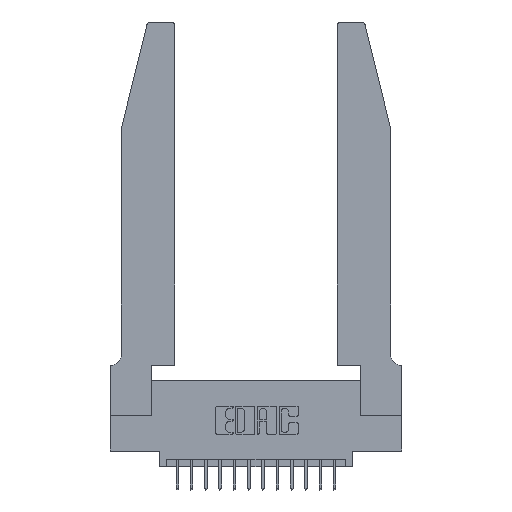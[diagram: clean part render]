
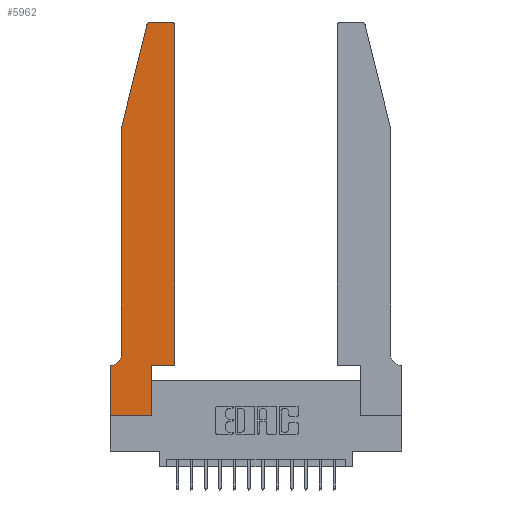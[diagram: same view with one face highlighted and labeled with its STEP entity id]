
A CAD part, top view. The second image highlights one B-rep face of the part: STEP entity #5962.
In plain terms, the highlighted planar face has unit normal (0, 0, 1).
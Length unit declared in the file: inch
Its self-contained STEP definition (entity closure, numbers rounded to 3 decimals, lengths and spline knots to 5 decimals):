
#3 = EDGE_CURVE ( 'NONE', #927, #10412, #13001, .T. ) ;
#71 = LINE ( 'NONE', #13692, #7374 ) ;
#250 = DIRECTION ( 'NONE',  ( -1., 0., 0. ) ) ;
#412 = DIRECTION ( 'NONE',  ( 0., 0., -1. ) ) ;
#456 = CARTESIAN_POINT ( 'NONE',  ( 0.0055, 0.42, 0.37 ) ) ;
#556 = VERTEX_POINT ( 'NONE', #3876 ) ;
#640 = EDGE_CURVE ( 'NONE', #1668, #1718, #12131, .T. ) ;
#649 = EDGE_CURVE ( 'NONE', #17177, #1668, #7938, .T. ) ;
#922 = CARTESIAN_POINT ( 'NONE',  ( 0., 0., 0.37 ) ) ;
#927 = VERTEX_POINT ( 'NONE', #11344 ) ;
#1026 = DIRECTION ( 'NONE',  ( -1., 0., 0. ) ) ;
#1089 = CARTESIAN_POINT ( 'NONE',  ( 0., 0.35, 0.37 ) ) ;
#1152 = DIRECTION ( 'NONE',  ( 0., 0., 1. ) ) ;
#1304 = CARTESIAN_POINT ( 'NONE',  ( 0.0755, 0.35, 0.37 ) ) ;
#1549 = CARTESIAN_POINT ( 'NONE',  ( 0.0755, 2., 0.37 ) ) ;
#1668 = VERTEX_POINT ( 'NONE', #14255 ) ;
#1718 = VERTEX_POINT ( 'NONE', #6900 ) ;
#1866 = VERTEX_POINT ( 'NONE', #14959 ) ;
#2091 = EDGE_CURVE ( 'NONE', #1866, #927, #12076, .T. ) ;
#2913 = DIRECTION ( 'NONE',  ( 0., 1., 0. ) ) ;
#3102 = CARTESIAN_POINT ( 'NONE',  ( 0., 0., 0.37 ) ) ;
#3514 = EDGE_CURVE ( 'NONE', #12185, #1866, #71, .T. ) ;
#3642 = ORIENTED_EDGE ( 'NONE', *, *, #7171, .T. ) ;
#3876 = CARTESIAN_POINT ( 'NONE',  ( 0.4505, 0.35, 0.37 ) ) ;
#4628 = ORIENTED_EDGE ( 'NONE', *, *, #11684, .T. ) ;
#4756 = EDGE_CURVE ( 'NONE', #1718, #15745, #13558, .T. ) ;
#4977 = LINE ( 'NONE', #10112, #15833 ) ;
#5350 = DIRECTION ( 'NONE',  ( 1., 0., 0. ) ) ;
#5507 = CARTESIAN_POINT ( 'NONE',  ( 0.4505, 2.72, 0.37 ) ) ;
#5734 = ORIENTED_EDGE ( 'NONE', *, *, #9515, .T. ) ;
#5784 = CARTESIAN_POINT ( 'NONE',  ( 0.4205, 2.75, 0.37 ) ) ;
#5852 = ORIENTED_EDGE ( 'NONE', *, *, #12724, .T. ) ;
#5944 = LINE ( 'NONE', #8941, #13019 ) ;
#5962 = ADVANCED_FACE ( 'NONE', ( #10022 ), #18184, .T. ) ;
#6038 = EDGE_CURVE ( 'NONE', #9966, #12185, #16599, .T. ) ;
#6865 = DIRECTION ( 'NONE',  ( 0., -1., 0. ) ) ;
#6900 = CARTESIAN_POINT ( 'NONE',  ( 0., 0.35, 0.37 ) ) ;
#7030 = LINE ( 'NONE', #15421, #17355 ) ;
#7051 = VERTEX_POINT ( 'NONE', #17083 ) ;
#7156 = DIRECTION ( 'NONE',  ( 0., 0., 1. ) ) ;
#7171 = EDGE_CURVE ( 'NONE', #7051, #556, #5944, .T. ) ;
#7374 = VECTOR ( 'NONE', #13710, 39.37008 ) ;
#7423 = LINE ( 'NONE', #12485, #11196 ) ;
#7938 = CIRCLE ( 'NONE', #14756, 0.07 ) ;
#8241 = ORIENTED_EDGE ( 'NONE', *, *, #9411, .T. ) ;
#8376 = DIRECTION ( 'NONE',  ( 0., 0., 1. ) ) ;
#8402 = CARTESIAN_POINT ( 'NONE',  ( 0.284, 2.72, 0.37 ) ) ;
#8458 = CARTESIAN_POINT ( 'NONE',  ( 0.0755, 0.42, 0.37 ) ) ;
#8479 = DIRECTION ( 'NONE',  ( 0., 1., 0. ) ) ;
#8941 = CARTESIAN_POINT ( 'NONE',  ( 0.4505, 0.35, 0.37 ) ) ;
#9255 = ORIENTED_EDGE ( 'NONE', *, *, #3, .T. ) ;
#9312 = VECTOR ( 'NONE', #13814, 39.37008 ) ;
#9331 = DIRECTION ( 'NONE',  ( 1., 0., 0. ) ) ;
#9411 = EDGE_CURVE ( 'NONE', #15745, #18095, #12546, .T. ) ;
#9515 = EDGE_CURVE ( 'NONE', #18095, #7051, #7030, .T. ) ;
#9784 = ORIENTED_EDGE ( 'NONE', *, *, #640, .T. ) ;
#9851 = VECTOR ( 'NONE', #11282, 39.37008 ) ;
#9876 = CARTESIAN_POINT ( 'NONE',  ( 0., 0., 0.37 ) ) ;
#9966 = VERTEX_POINT ( 'NONE', #5507 ) ;
#10022 = FACE_OUTER_BOUND ( 'NONE', #18165, .T. ) ;
#10087 = AXIS2_PLACEMENT_3D ( 'NONE', #1089, #1152, #11244 ) ;
#10112 = CARTESIAN_POINT ( 'NONE',  ( 0.4505, 0.35, 0.37 ) ) ;
#10353 = DIRECTION ( 'NONE',  ( 1., 0., 0. ) ) ;
#10412 = VERTEX_POINT ( 'NONE', #15215 ) ;
#11041 = AXIS2_PLACEMENT_3D ( 'NONE', #15589, #7156, #16990 ) ;
#11196 = VECTOR ( 'NONE', #6865, 39.37008 ) ;
#11244 = DIRECTION ( 'NONE',  ( 1., 0., 0. ) ) ;
#11282 = DIRECTION ( 'NONE',  ( 0., -1., 0. ) ) ;
#11344 = CARTESIAN_POINT ( 'NONE',  ( 0.25487, 2.72718, 0.37 ) ) ;
#11670 = VECTOR ( 'NONE', #5350, 39.37008 ) ;
#11684 = EDGE_CURVE ( 'NONE', #556, #9966, #4977, .T. ) ;
#12076 = CIRCLE ( 'NONE', #15242, 0.03 ) ;
#12131 = LINE ( 'NONE', #1304, #15420 ) ;
#12185 = VERTEX_POINT ( 'NONE', #5784 ) ;
#12485 = CARTESIAN_POINT ( 'NONE',  ( 0.0755, 2., 0.37 ) ) ;
#12546 = LINE ( 'NONE', #922, #11670 ) ;
#12724 = EDGE_CURVE ( 'NONE', #10412, #17177, #7423, .T. ) ;
#13001 = LINE ( 'NONE', #1549, #9312 ) ;
#13019 = VECTOR ( 'NONE', #10353, 39.37008 ) ;
#13203 = ORIENTED_EDGE ( 'NONE', *, *, #4756, .T. ) ;
#13558 = LINE ( 'NONE', #9876, #9851 ) ;
#13692 = CARTESIAN_POINT ( 'NONE',  ( 0.2605, 2.75, 0.37 ) ) ;
#13710 = DIRECTION ( 'NONE',  ( -1., 0., 0. ) ) ;
#13814 = DIRECTION ( 'NONE',  ( -0.239, -0.971, 0. ) ) ;
#14062 = ORIENTED_EDGE ( 'NONE', *, *, #3514, .T. ) ;
#14255 = CARTESIAN_POINT ( 'NONE',  ( 0.0055, 0.35, 0.37 ) ) ;
#14756 = AXIS2_PLACEMENT_3D ( 'NONE', #456, #412, #250 ) ;
#14959 = CARTESIAN_POINT ( 'NONE',  ( 0.284, 2.75, 0.37 ) ) ;
#15215 = CARTESIAN_POINT ( 'NONE',  ( 0.0755, 2., 0.37 ) ) ;
#15242 = AXIS2_PLACEMENT_3D ( 'NONE', #8402, #8376, #9331 ) ;
#15420 = VECTOR ( 'NONE', #1026, 39.37008 ) ;
#15421 = CARTESIAN_POINT ( 'NONE',  ( 0.2865, 0.35, 0.37 ) ) ;
#15589 = CARTESIAN_POINT ( 'NONE',  ( 0.4205, 2.72, 0.37 ) ) ;
#15745 = VERTEX_POINT ( 'NONE', #3102 ) ;
#15833 = VECTOR ( 'NONE', #2913, 39.37008 ) ;
#16084 = ORIENTED_EDGE ( 'NONE', *, *, #649, .T. ) ;
#16599 = CIRCLE ( 'NONE', #11041, 0.03 ) ;
#16990 = DIRECTION ( 'NONE',  ( 1., 0., 0. ) ) ;
#17036 = CARTESIAN_POINT ( 'NONE',  ( 0.2865, 0., 0.37 ) ) ;
#17083 = CARTESIAN_POINT ( 'NONE',  ( 0.2865, 0.35, 0.37 ) ) ;
#17131 = ORIENTED_EDGE ( 'NONE', *, *, #2091, .T. ) ;
#17177 = VERTEX_POINT ( 'NONE', #8458 ) ;
#17355 = VECTOR ( 'NONE', #8479, 39.37008 ) ;
#17701 = ORIENTED_EDGE ( 'NONE', *, *, #6038, .T. ) ;
#18095 = VERTEX_POINT ( 'NONE', #17036 ) ;
#18165 = EDGE_LOOP ( 'NONE', ( #14062, #17131, #9255, #5852, #16084, #9784, #13203, #8241, #5734, #3642, #4628, #17701 ) ) ;
#18184 = PLANE ( 'NONE',  #10087 ) ;
